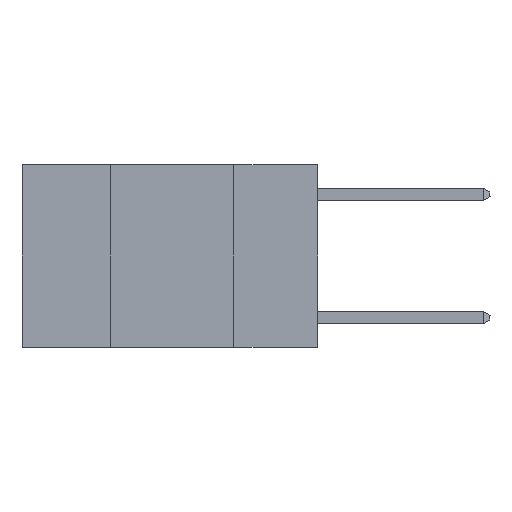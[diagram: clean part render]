
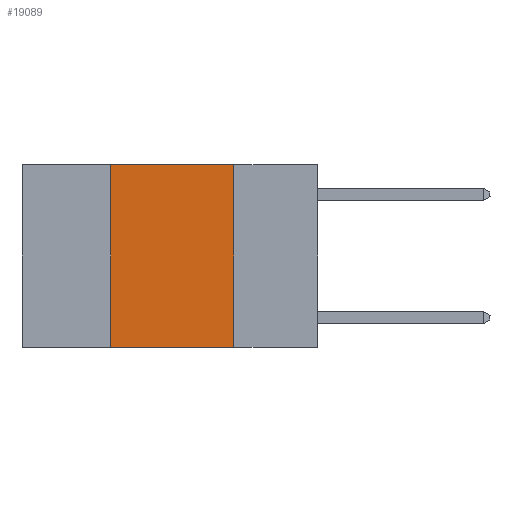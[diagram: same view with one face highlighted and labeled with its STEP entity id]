
A CAD part, left-side view. The second image highlights one B-rep face of the part: STEP entity #19089.
In plain terms, the highlighted planar face has unit normal (-1, 0, 0).
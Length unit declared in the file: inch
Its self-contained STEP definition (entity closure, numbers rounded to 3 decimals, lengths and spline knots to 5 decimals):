
#1105 = EDGE_CURVE ( 'NONE', #4010, #23492, #10884, .T. ) ;
#2134 = VECTOR ( 'NONE', #17177, 39.37008 ) ;
#2455 = ORIENTED_EDGE ( 'NONE', *, *, #8260, .T. ) ;
#3012 = CARTESIAN_POINT ( 'NONE',  ( 0., 0.42, -0.37 ) ) ;
#3074 = VECTOR ( 'NONE', #3357, 39.37008 ) ;
#3357 = DIRECTION ( 'NONE',  ( 0., 0., -1. ) ) ;
#3836 = LINE ( 'NONE', #11877, #2134 ) ;
#3928 = ORIENTED_EDGE ( 'NONE', *, *, #1105, .F. ) ;
#4010 = VERTEX_POINT ( 'NONE', #11136 ) ;
#5320 = CARTESIAN_POINT ( 'NONE',  ( 0., 0.17, 0. ) ) ;
#5852 = LINE ( 'NONE', #11565, #22956 ) ;
#6969 = VERTEX_POINT ( 'NONE', #3012 ) ;
#7127 = CARTESIAN_POINT ( 'NONE',  ( 0., 0.6, 0. ) ) ;
#7376 = DIRECTION ( 'NONE',  ( 0., 0., -1. ) ) ;
#8260 = EDGE_CURVE ( 'NONE', #6969, #23492, #5852, .T. ) ;
#8881 = FACE_OUTER_BOUND ( 'NONE', #13494, .T. ) ;
#10884 = LINE ( 'NONE', #5320, #3074 ) ;
#11136 = CARTESIAN_POINT ( 'NONE',  ( 0., 0.17, 0. ) ) ;
#11565 = CARTESIAN_POINT ( 'NONE',  ( 0., 0.6, -0.37 ) ) ;
#11877 = CARTESIAN_POINT ( 'NONE',  ( 0., 0.6, 0. ) ) ;
#12051 = VECTOR ( 'NONE', #19702, 39.37008 ) ;
#13252 = VERTEX_POINT ( 'NONE', #22506 ) ;
#13310 = EDGE_CURVE ( 'NONE', #13252, #4010, #3836, .T. ) ;
#13494 = EDGE_LOOP ( 'NONE', ( #3928, #16949, #17202, #2455 ) ) ;
#14006 = LINE ( 'NONE', #22259, #12051 ) ;
#15476 = DIRECTION ( 'NONE',  ( 0., -1., 0. ) ) ;
#15577 = CARTESIAN_POINT ( 'NONE',  ( 0., 0.17, -0.37 ) ) ;
#16428 = PLANE ( 'NONE',  #21543 ) ;
#16949 = ORIENTED_EDGE ( 'NONE', *, *, #13310, .F. ) ;
#17076 = EDGE_CURVE ( 'NONE', #6969, #13252, #14006, .T. ) ;
#17177 = DIRECTION ( 'NONE',  ( 0., -1., 0. ) ) ;
#17202 = ORIENTED_EDGE ( 'NONE', *, *, #17076, .F. ) ;
#19089 = ADVANCED_FACE ( 'NONE', ( #8881 ), #16428, .F. ) ;
#19702 = DIRECTION ( 'NONE',  ( 0., 0., 1. ) ) ;
#21543 = AXIS2_PLACEMENT_3D ( 'NONE', #7127, #22267, #7376 ) ;
#22259 = CARTESIAN_POINT ( 'NONE',  ( 0., 0.42, 0. ) ) ;
#22267 = DIRECTION ( 'NONE',  ( 1., 0., 0. ) ) ;
#22506 = CARTESIAN_POINT ( 'NONE',  ( 0., 0.42, 0. ) ) ;
#22956 = VECTOR ( 'NONE', #15476, 39.37008 ) ;
#23492 = VERTEX_POINT ( 'NONE', #15577 ) ;
